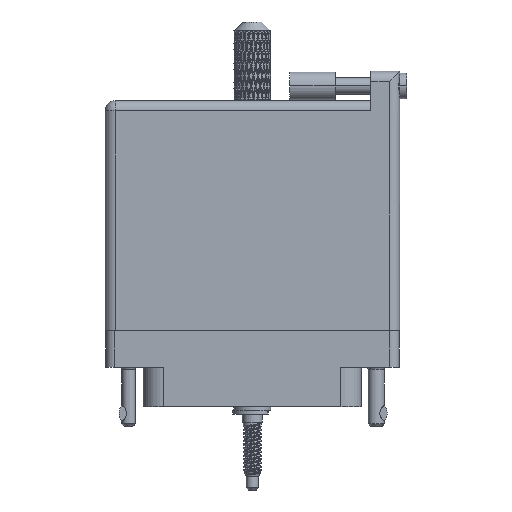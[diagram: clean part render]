
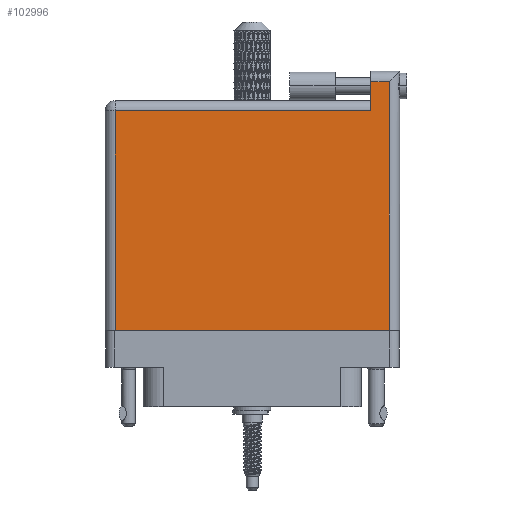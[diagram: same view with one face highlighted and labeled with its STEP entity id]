
A CAD part, front view. The second image highlights one B-rep face of the part: STEP entity #102996.
In plain terms, the highlighted face is planar.
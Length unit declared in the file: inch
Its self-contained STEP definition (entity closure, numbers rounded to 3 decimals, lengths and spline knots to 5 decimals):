
#2843 = CARTESIAN_POINT ( 'NONE',  ( 0.807, 1.396, 0.4495 ) ) ;
#7110 = CARTESIAN_POINT ( 'NONE',  ( 0.807, 1.596, 0.4495 ) ) ;
#7124 = AXIS2_PLACEMENT_3D ( 'NONE', #28965, #37882, #20425 ) ;
#13856 = LINE ( 'NONE', #25080, #63815 ) ;
#20425 = DIRECTION ( 'NONE',  ( -1., 0., 0. ) ) ;
#21046 = VECTOR ( 'NONE', #93681, 39.37008 ) ;
#23909 = VERTEX_POINT ( 'NONE', #7110 ) ;
#24023 = CARTESIAN_POINT ( 'NONE',  ( -0.934, -0.1, 0.4495 ) ) ;
#25080 = CARTESIAN_POINT ( 'NONE',  ( -0.934, -0.1, 0.4495 ) ) ;
#26128 = LINE ( 'NONE', #44223, #90022 ) ;
#27235 = LINE ( 'NONE', #42845, #99369 ) ;
#28965 = CARTESIAN_POINT ( 'NONE',  ( -1.004, 1.466, 0.4495 ) ) ;
#30018 = EDGE_CURVE ( 'NONE', #68130, #23909, #98877, .T. ) ;
#32223 = VERTEX_POINT ( 'NONE', #73449 ) ;
#34875 = CARTESIAN_POINT ( 'NONE',  ( -1.004, 1.596, 0.4495 ) ) ;
#35133 = VERTEX_POINT ( 'NONE', #2843 ) ;
#35603 = CARTESIAN_POINT ( 'NONE',  ( -0.934, 1.396, 0.4495 ) ) ;
#36737 = PLANE ( 'NONE',  #7124 ) ;
#37882 = DIRECTION ( 'NONE',  ( 0., 0., -1. ) ) ;
#38967 = FACE_OUTER_BOUND ( 'NONE', #92138, .T. ) ;
#42845 = CARTESIAN_POINT ( 'NONE',  ( -1.004, 1.396, 0.4495 ) ) ;
#43197 = CARTESIAN_POINT ( 'NONE',  ( 0.807, 1.666, 0.4495 ) ) ;
#43555 = EDGE_CURVE ( 'NONE', #69560, #32223, #26128, .T. ) ;
#44223 = CARTESIAN_POINT ( 'NONE',  ( -1.004, -0.1, 0.4495 ) ) ;
#46222 = EDGE_CURVE ( 'NONE', #35133, #58917, #27235, .T. ) ;
#46914 = ORIENTED_EDGE ( 'NONE', *, *, #43555, .T. ) ;
#51725 = VECTOR ( 'NONE', #78741, 39.37008 ) ;
#53699 = ORIENTED_EDGE ( 'NONE', *, *, #72725, .T. ) ;
#55309 = CARTESIAN_POINT ( 'NONE',  ( 0.934, 1.666, 0.4495 ) ) ;
#56183 = EDGE_CURVE ( 'NONE', #32223, #68130, #87606, .T. ) ;
#58917 = VERTEX_POINT ( 'NONE', #35603 ) ;
#62053 = DIRECTION ( 'NONE',  ( 1., 0., 0. ) ) ;
#63815 = VECTOR ( 'NONE', #70472, 39.37008 ) ;
#68130 = VERTEX_POINT ( 'NONE', #104884 ) ;
#69560 = VERTEX_POINT ( 'NONE', #24023 ) ;
#70472 = DIRECTION ( 'NONE',  ( 0., -1., 0. ) ) ;
#71916 = LINE ( 'NONE', #43197, #98290 ) ;
#72725 = EDGE_CURVE ( 'NONE', #58917, #69560, #13856, .T. ) ;
#73449 = CARTESIAN_POINT ( 'NONE',  ( 0.934, -0.1, 0.4495 ) ) ;
#77699 = DIRECTION ( 'NONE',  ( 0., -1., 0. ) ) ;
#78741 = DIRECTION ( 'NONE',  ( -1., 0., 0. ) ) ;
#87606 = LINE ( 'NONE', #55309, #21046 ) ;
#88491 = EDGE_CURVE ( 'NONE', #23909, #35133, #71916, .T. ) ;
#90022 = VECTOR ( 'NONE', #62053, 39.37008 ) ;
#92138 = EDGE_LOOP ( 'NONE', ( #46914, #98608, #98327, #110259, #113618, #53699 ) ) ;
#93681 = DIRECTION ( 'NONE',  ( 0., 1., 0. ) ) ;
#98290 = VECTOR ( 'NONE', #77699, 39.37008 ) ;
#98327 = ORIENTED_EDGE ( 'NONE', *, *, #30018, .T. ) ;
#98608 = ORIENTED_EDGE ( 'NONE', *, *, #56183, .T. ) ;
#98877 = LINE ( 'NONE', #34875, #51725 ) ;
#99369 = VECTOR ( 'NONE', #113396, 39.37008 ) ;
#102996 = ADVANCED_FACE ( 'NONE', ( #38967 ), #36737, .F. ) ;
#104884 = CARTESIAN_POINT ( 'NONE',  ( 0.934, 1.596, 0.4495 ) ) ;
#110259 = ORIENTED_EDGE ( 'NONE', *, *, #88491, .T. ) ;
#113396 = DIRECTION ( 'NONE',  ( -1., 0., 0. ) ) ;
#113618 = ORIENTED_EDGE ( 'NONE', *, *, #46222, .T. ) ;
